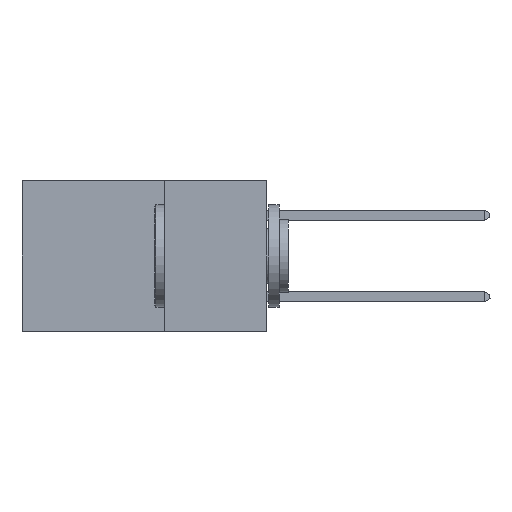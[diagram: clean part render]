
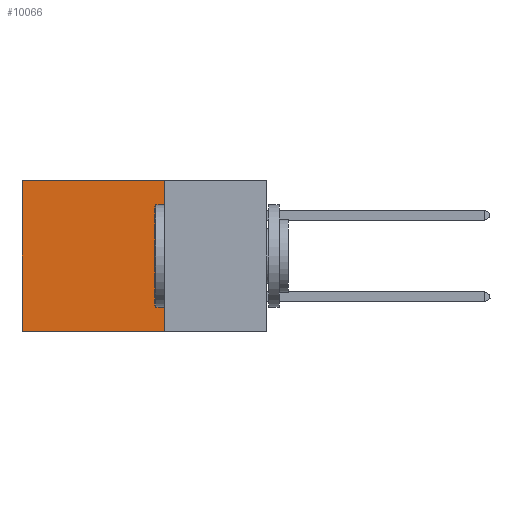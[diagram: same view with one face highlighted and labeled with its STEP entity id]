
A CAD part, left-side view. The second image highlights one B-rep face of the part: STEP entity #10066.
In plain terms, the highlighted planar face has unit normal (-1, 0, 0).
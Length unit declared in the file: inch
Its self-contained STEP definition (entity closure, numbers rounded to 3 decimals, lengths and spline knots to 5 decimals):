
#161 = LINE ( 'NONE', #3946, #20961 ) ;
#3901 = VERTEX_POINT ( 'NONE', #20307 ) ;
#3946 = CARTESIAN_POINT ( 'NONE',  ( 0.2875, 0.6, 0. ) ) ;
#5599 = DIRECTION ( 'NONE',  ( 0., 1., 0. ) ) ;
#6035 = CARTESIAN_POINT ( 'NONE',  ( 0.2875, 0.25, -0.37 ) ) ;
#8385 = CARTESIAN_POINT ( 'NONE',  ( 0.2875, 0.25, 0. ) ) ;
#8426 = CARTESIAN_POINT ( 'NONE',  ( 0.2875, 0.25, 0. ) ) ;
#9542 = ORIENTED_EDGE ( 'NONE', *, *, #14228, .T. ) ;
#10066 = ADVANCED_FACE ( 'NONE', ( #13898 ), #21607, .F. ) ;
#13857 = CARTESIAN_POINT ( 'NONE',  ( 0.2875, 0.25, -0.37 ) ) ;
#13898 = FACE_OUTER_BOUND ( 'NONE', #26920, .T. ) ;
#14228 = EDGE_CURVE ( 'NONE', #3901, #24070, #161, .T. ) ;
#16770 = EDGE_CURVE ( 'NONE', #40294, #24070, #33967, .T. ) ;
#17724 = LINE ( 'NONE', #26770, #29004 ) ;
#20307 = CARTESIAN_POINT ( 'NONE',  ( 0.2875, 0.6, 0. ) ) ;
#20726 = VECTOR ( 'NONE', #5599, 39.37008 ) ;
#20799 = EDGE_CURVE ( 'NONE', #38733, #3901, #25277, .T. ) ;
#20961 = VECTOR ( 'NONE', #39992, 39.37008 ) ;
#21295 = DIRECTION ( 'NONE',  ( 0., 1., 0. ) ) ;
#21607 = PLANE ( 'NONE',  #38842 ) ;
#22110 = ORIENTED_EDGE ( 'NONE', *, *, #20799, .T. ) ;
#24070 = VERTEX_POINT ( 'NONE', #41605 ) ;
#24893 = DIRECTION ( 'NONE',  ( 0., 0., -1. ) ) ;
#25277 = LINE ( 'NONE', #8385, #32945 ) ;
#26570 = ORIENTED_EDGE ( 'NONE', *, *, #35178, .F. ) ;
#26695 = ORIENTED_EDGE ( 'NONE', *, *, #16770, .F. ) ;
#26770 = CARTESIAN_POINT ( 'NONE',  ( 0.2875, 0.25, 0. ) ) ;
#26920 = EDGE_LOOP ( 'NONE', ( #9542, #26695, #26570, #22110 ) ) ;
#29004 = VECTOR ( 'NONE', #39528, 39.37008 ) ;
#32945 = VECTOR ( 'NONE', #21295, 39.37008 ) ;
#33967 = LINE ( 'NONE', #6035, #20726 ) ;
#35178 = EDGE_CURVE ( 'NONE', #38733, #40294, #17724, .T. ) ;
#37973 = DIRECTION ( 'NONE',  ( 1., 0., 0. ) ) ;
#38733 = VERTEX_POINT ( 'NONE', #41400 ) ;
#38842 = AXIS2_PLACEMENT_3D ( 'NONE', #8426, #37973, #24893 ) ;
#39528 = DIRECTION ( 'NONE',  ( 0., 0., -1. ) ) ;
#39992 = DIRECTION ( 'NONE',  ( 0., 0., -1. ) ) ;
#40294 = VERTEX_POINT ( 'NONE', #13857 ) ;
#41400 = CARTESIAN_POINT ( 'NONE',  ( 0.2875, 0.25, 0. ) ) ;
#41605 = CARTESIAN_POINT ( 'NONE',  ( 0.2875, 0.6, -0.37 ) ) ;
